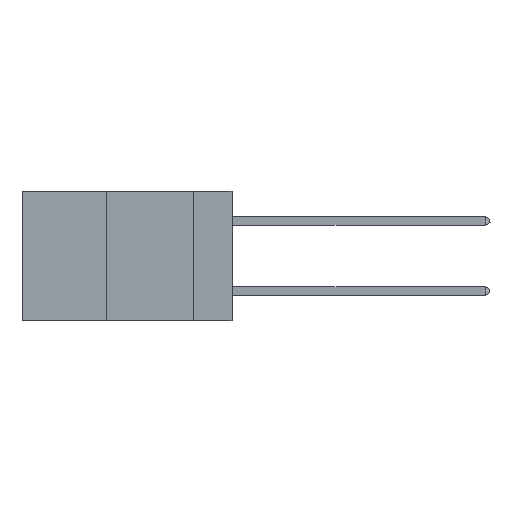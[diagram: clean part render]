
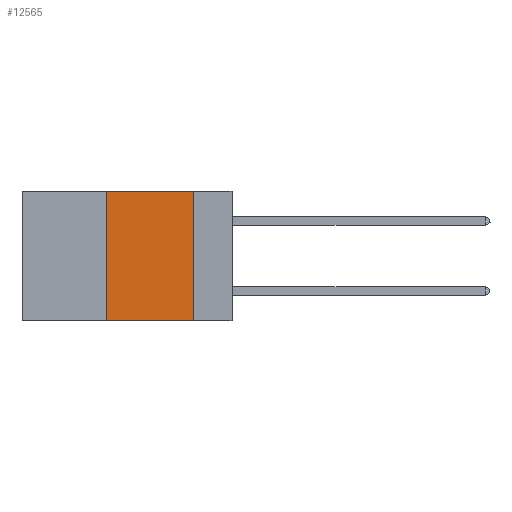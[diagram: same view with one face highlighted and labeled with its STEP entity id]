
A CAD part, left-side view. The second image highlights one B-rep face of the part: STEP entity #12565.
In plain terms, the highlighted planar face has unit normal (-1, 0, 0).
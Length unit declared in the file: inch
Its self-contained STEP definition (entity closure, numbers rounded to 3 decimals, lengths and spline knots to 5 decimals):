
#368 = CARTESIAN_POINT ( 'NONE',  ( 0., 0.36, 0. ) ) ;
#768 = DIRECTION ( 'NONE',  ( 0., -1., 0. ) ) ;
#2110 = EDGE_CURVE ( 'NONE', #3140, #21370, #13393, .T. ) ;
#3140 = VERTEX_POINT ( 'NONE', #368 ) ;
#3591 = DIRECTION ( 'NONE',  ( 0., 0., -1. ) ) ;
#3845 = CARTESIAN_POINT ( 'NONE',  ( 0., 0.11, 0. ) ) ;
#4089 = VECTOR ( 'NONE', #768, 39.37008 ) ;
#5184 = FACE_OUTER_BOUND ( 'NONE', #22375, .T. ) ;
#5442 = CARTESIAN_POINT ( 'NONE',  ( 0., 0.36, 0. ) ) ;
#5702 = LINE ( 'NONE', #5442, #6630 ) ;
#6175 = CARTESIAN_POINT ( 'NONE',  ( 0., 0.6, 0. ) ) ;
#6630 = VECTOR ( 'NONE', #15462, 39.37008 ) ;
#6896 = CARTESIAN_POINT ( 'NONE',  ( 0., 0.36, -0.37 ) ) ;
#8168 = DIRECTION ( 'NONE',  ( 0., 0., -1. ) ) ;
#8309 = CARTESIAN_POINT ( 'NONE',  ( 0., 0.6, 0. ) ) ;
#8647 = LINE ( 'NONE', #18674, #19576 ) ;
#10695 = ORIENTED_EDGE ( 'NONE', *, *, #19136, .T. ) ;
#10737 = EDGE_CURVE ( 'NONE', #21370, #21371, #20609, .T. ) ;
#12565 = ADVANCED_FACE ( 'NONE', ( #5184 ), #24059, .F. ) ;
#12731 = VECTOR ( 'NONE', #3591, 39.37008 ) ;
#13393 = LINE ( 'NONE', #8309, #4089 ) ;
#13744 = CARTESIAN_POINT ( 'NONE',  ( 0., 0.11, -0.37 ) ) ;
#14166 = DIRECTION ( 'NONE',  ( 1., 0., 0. ) ) ;
#14386 = DIRECTION ( 'NONE',  ( 0., -1., 0. ) ) ;
#15075 = ORIENTED_EDGE ( 'NONE', *, *, #10737, .F. ) ;
#15366 = EDGE_CURVE ( 'NONE', #19363, #3140, #5702, .T. ) ;
#15462 = DIRECTION ( 'NONE',  ( 0., 0., 1. ) ) ;
#16028 = ORIENTED_EDGE ( 'NONE', *, *, #2110, .F. ) ;
#18674 = CARTESIAN_POINT ( 'NONE',  ( 0., 0.6, -0.37 ) ) ;
#19136 = EDGE_CURVE ( 'NONE', #19363, #21371, #8647, .T. ) ;
#19363 = VERTEX_POINT ( 'NONE', #6896 ) ;
#19535 = CARTESIAN_POINT ( 'NONE',  ( 0., 0.11, 0. ) ) ;
#19576 = VECTOR ( 'NONE', #14386, 39.37008 ) ;
#20609 = LINE ( 'NONE', #19535, #12731 ) ;
#21370 = VERTEX_POINT ( 'NONE', #3845 ) ;
#21371 = VERTEX_POINT ( 'NONE', #13744 ) ;
#21550 = AXIS2_PLACEMENT_3D ( 'NONE', #6175, #14166, #8168 ) ;
#22375 = EDGE_LOOP ( 'NONE', ( #15075, #16028, #23513, #10695 ) ) ;
#23513 = ORIENTED_EDGE ( 'NONE', *, *, #15366, .F. ) ;
#24059 = PLANE ( 'NONE',  #21550 ) ;
